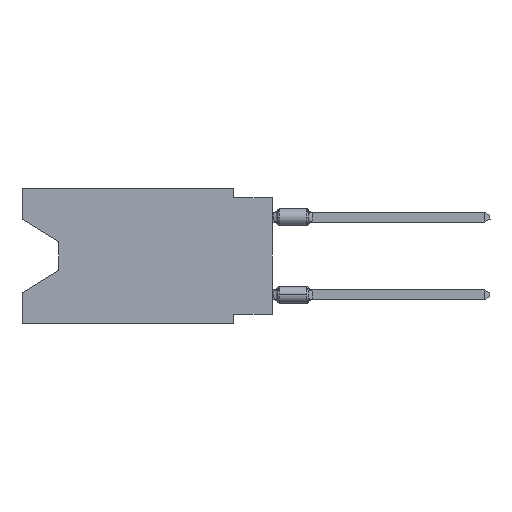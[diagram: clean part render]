
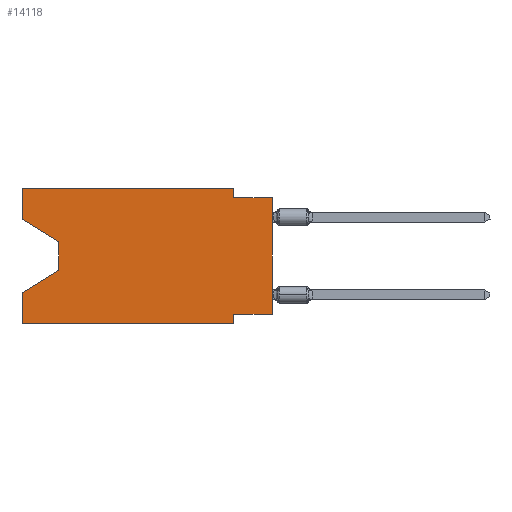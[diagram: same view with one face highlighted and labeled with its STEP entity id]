
A CAD part, left-side view. The second image highlights one B-rep face of the part: STEP entity #14118.
In plain terms, the highlighted planar face has unit normal (-1, 0, 0).
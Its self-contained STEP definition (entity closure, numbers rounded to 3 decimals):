
#456 = CARTESIAN_POINT ( 'NONE',  ( 0., 16.383, 0. ) ) ;
#830 = FACE_OUTER_BOUND ( 'NONE', #5389, .T. ) ;
#1389 = VECTOR ( 'NONE', #18368, 1000. ) ;
#1504 = VECTOR ( 'NONE', #3200, 1000. ) ;
#1713 = VERTEX_POINT ( 'NONE', #45329 ) ;
#2420 = DIRECTION ( 'NONE',  ( 0., 0., 1. ) ) ;
#2847 = ORIENTED_EDGE ( 'NONE', *, *, #6545, .T. ) ;
#3200 = DIRECTION ( 'NONE',  ( 0., 0., -1. ) ) ;
#3350 = ORIENTED_EDGE ( 'NONE', *, *, #25113, .F. ) ;
#5119 = VECTOR ( 'NONE', #28029, 1000. ) ;
#5389 = EDGE_LOOP ( 'NONE', ( #43956, #43417, #31614, #21980, #39325, #15211, #22337, #2847, #3350, #44732, #7300, #25105 ) ) ;
#6111 = VECTOR ( 'NONE', #31538, 1000. ) ;
#6545 = EDGE_CURVE ( 'NONE', #36232, #38671, #42025, .T. ) ;
#6789 = CARTESIAN_POINT ( 'NONE',  ( 0., 0., -0.635 ) ) ;
#7300 = ORIENTED_EDGE ( 'NONE', *, *, #16772, .F. ) ;
#7908 = CARTESIAN_POINT ( 'NONE',  ( 0., 13.97, -3.505 ) ) ;
#9099 = EDGE_CURVE ( 'NONE', #31616, #31832, #25893, .T. ) ;
#9179 = AXIS2_PLACEMENT_3D ( 'NONE', #31583, #15939, #26873 ) ;
#9463 = VECTOR ( 'NONE', #15192, 1000. ) ;
#9967 = CARTESIAN_POINT ( 'NONE',  ( 0., 0., -8.255 ) ) ;
#10752 = EDGE_CURVE ( 'NONE', #40222, #1713, #22348, .T. ) ;
#10836 = EDGE_CURVE ( 'NONE', #16464, #12461, #20378, .T. ) ;
#11095 = EDGE_CURVE ( 'NONE', #36076, #40222, #37185, .T. ) ;
#11821 = LINE ( 'NONE', #46332, #32078 ) ;
#11853 = LINE ( 'NONE', #45623, #15240 ) ;
#12461 = VERTEX_POINT ( 'NONE', #36532 ) ;
#14118 = ADVANCED_FACE ( 'NONE', ( #830 ), #38799, .F. ) ;
#14222 = EDGE_CURVE ( 'NONE', #36232, #42773, #16684, .T. ) ;
#15192 = DIRECTION ( 'NONE',  ( 0., 0., -1. ) ) ;
#15211 = ORIENTED_EDGE ( 'NONE', *, *, #43907, .F. ) ;
#15240 = VECTOR ( 'NONE', #41619, 1000. ) ;
#15939 = DIRECTION ( 'NONE',  ( 1., 0., 0. ) ) ;
#16330 = VECTOR ( 'NONE', #25104, 1000. ) ;
#16383 = LINE ( 'NONE', #16625, #5119 ) ;
#16464 = VERTEX_POINT ( 'NONE', #23931 ) ;
#16535 = DIRECTION ( 'NONE',  ( 0., 0., 1. ) ) ;
#16625 = CARTESIAN_POINT ( 'NONE',  ( 0., 2.54, -8.89 ) ) ;
#16684 = LINE ( 'NONE', #9967, #16330 ) ;
#16772 = EDGE_CURVE ( 'NONE', #25617, #31616, #11853, .T. ) ;
#18368 = DIRECTION ( 'NONE',  ( 0., 0.855, -0.519 ) ) ;
#19255 = EDGE_CURVE ( 'NONE', #34437, #25617, #43612, .T. ) ;
#19277 = VECTOR ( 'NONE', #2420, 1000. ) ;
#20197 = VECTOR ( 'NONE', #16535, 1000. ) ;
#20378 = LINE ( 'NONE', #27323, #6111 ) ;
#21143 = CARTESIAN_POINT ( 'NONE',  ( 0., 13.97, -3.505 ) ) ;
#21980 = ORIENTED_EDGE ( 'NONE', *, *, #37799, .F. ) ;
#22337 = ORIENTED_EDGE ( 'NONE', *, *, #14222, .F. ) ;
#22348 = LINE ( 'NONE', #48694, #1389 ) ;
#22383 = DIRECTION ( 'NONE',  ( 0., -1., 0. ) ) ;
#23931 = CARTESIAN_POINT ( 'NONE',  ( 0., 16.383, -8.89 ) ) ;
#25104 = DIRECTION ( 'NONE',  ( 0., 1., 0. ) ) ;
#25105 = ORIENTED_EDGE ( 'NONE', *, *, #19255, .F. ) ;
#25113 = EDGE_CURVE ( 'NONE', #31832, #38671, #37274, .T. ) ;
#25150 = VECTOR ( 'NONE', #27641, 1000. ) ;
#25476 = CARTESIAN_POINT ( 'NONE',  ( 0., 0., -0.635 ) ) ;
#25617 = VERTEX_POINT ( 'NONE', #456 ) ;
#25893 = LINE ( 'NONE', #26880, #9463 ) ;
#25989 = VECTOR ( 'NONE', #22383, 1000. ) ;
#26873 = DIRECTION ( 'NONE',  ( 0., 0., -1. ) ) ;
#26880 = CARTESIAN_POINT ( 'NONE',  ( 0., 2.54, 0. ) ) ;
#27323 = CARTESIAN_POINT ( 'NONE',  ( 0., 16.383, -8.89 ) ) ;
#27641 = DIRECTION ( 'NONE',  ( 0., 0., 1. ) ) ;
#28019 = CARTESIAN_POINT ( 'NONE',  ( 0., 2.54, -8.255 ) ) ;
#28029 = DIRECTION ( 'NONE',  ( 0., 0., -1. ) ) ;
#31093 = CARTESIAN_POINT ( 'NONE',  ( 0., 0., 0. ) ) ;
#31538 = DIRECTION ( 'NONE',  ( 0., -1., 0. ) ) ;
#31583 = CARTESIAN_POINT ( 'NONE',  ( 0., 16.383, 0. ) ) ;
#31614 = ORIENTED_EDGE ( 'NONE', *, *, #10752, .T. ) ;
#31616 = VERTEX_POINT ( 'NONE', #45768 ) ;
#31832 = VERTEX_POINT ( 'NONE', #46981 ) ;
#32078 = VECTOR ( 'NONE', #42835, 1000. ) ;
#32387 = CARTESIAN_POINT ( 'NONE',  ( 0., 16.383, 0. ) ) ;
#34437 = VERTEX_POINT ( 'NONE', #36080 ) ;
#35878 = CARTESIAN_POINT ( 'NONE',  ( 0., 13.97, -5.385 ) ) ;
#36076 = VERTEX_POINT ( 'NONE', #21143 ) ;
#36080 = CARTESIAN_POINT ( 'NONE',  ( 0., 16.383, -2.038 ) ) ;
#36232 = VERTEX_POINT ( 'NONE', #37464 ) ;
#36532 = CARTESIAN_POINT ( 'NONE',  ( 0., 2.54, -8.89 ) ) ;
#37185 = LINE ( 'NONE', #7908, #1504 ) ;
#37274 = LINE ( 'NONE', #6789, #25989 ) ;
#37464 = CARTESIAN_POINT ( 'NONE',  ( 0., 0., -8.255 ) ) ;
#37615 = EDGE_CURVE ( 'NONE', #34437, #36076, #11821, .T. ) ;
#37799 = EDGE_CURVE ( 'NONE', #16464, #1713, #47558, .T. ) ;
#38671 = VERTEX_POINT ( 'NONE', #25476 ) ;
#38799 = PLANE ( 'NONE',  #9179 ) ;
#39325 = ORIENTED_EDGE ( 'NONE', *, *, #10836, .T. ) ;
#40145 = CARTESIAN_POINT ( 'NONE',  ( 0., 16.383, 0. ) ) ;
#40222 = VERTEX_POINT ( 'NONE', #35878 ) ;
#41619 = DIRECTION ( 'NONE',  ( 0., -1., 0. ) ) ;
#42025 = LINE ( 'NONE', #31093, #25150 ) ;
#42773 = VERTEX_POINT ( 'NONE', #28019 ) ;
#42835 = DIRECTION ( 'NONE',  ( 0., -0.855, -0.519 ) ) ;
#43417 = ORIENTED_EDGE ( 'NONE', *, *, #11095, .T. ) ;
#43612 = LINE ( 'NONE', #40145, #19277 ) ;
#43907 = EDGE_CURVE ( 'NONE', #42773, #12461, #16383, .T. ) ;
#43956 = ORIENTED_EDGE ( 'NONE', *, *, #37615, .T. ) ;
#44732 = ORIENTED_EDGE ( 'NONE', *, *, #9099, .F. ) ;
#45329 = CARTESIAN_POINT ( 'NONE',  ( 0., 16.383, -6.852 ) ) ;
#45623 = CARTESIAN_POINT ( 'NONE',  ( 0., 16.383, 0. ) ) ;
#45768 = CARTESIAN_POINT ( 'NONE',  ( 0., 2.54, 0. ) ) ;
#46332 = CARTESIAN_POINT ( 'NONE',  ( 0., 16.383, -2.038 ) ) ;
#46981 = CARTESIAN_POINT ( 'NONE',  ( 0., 2.54, -0.635 ) ) ;
#47558 = LINE ( 'NONE', #32387, #20197 ) ;
#48694 = CARTESIAN_POINT ( 'NONE',  ( 0., 13.97, -5.385 ) ) ;
